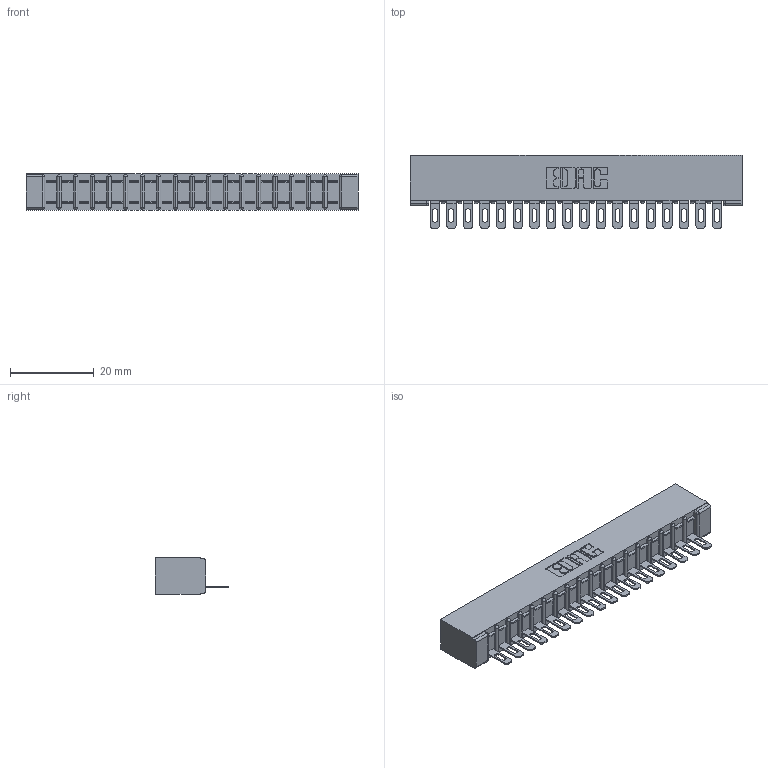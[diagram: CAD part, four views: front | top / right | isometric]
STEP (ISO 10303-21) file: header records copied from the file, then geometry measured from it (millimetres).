
FILE_DESCRIPTION (( 'STEP AP203' ), '1' );
FILE_NAME ('357-018-401-101.STEP', '2020-10-01T00:16:39', ( '' ), ( '' ), 'SwSTEP 2.0', 'SolidWorks 2020', '' );
FILE_SCHEMA (( 'CONFIG_CONTROL_DESIGN' ));
Length unit declared in the file: inch
Products named in the file (3): 357-018-401-101; 307-290-002_501; 307 Part_No Mounting Lugs
Assembly tree (19 placements, depth 2):
  357-018-401-101
    307 Part_No Mounting Lugs
    307-290-002_501  x18
Bounding box: 79.2 x 17.42 x 8.71 mm (x, y, z)
Volume: 5484.3 mm3; surface area: 10381.1 mm2
Topology: 19 solids, 19 shells, 1497 faces, 4583 edges, 3002 vertices
Faces by surface type: plane 858, cylinder 601, sphere 38
Entity records: 18906 total; most frequent: CARTESIAN_POINT 3184, ORIENTED_EDGE 3174, DIRECTION 3107, EDGE_CURVE 1587, VECTOR 1201, LINE 1201, VERTEX_POINT 1030, AXIS2_PLACEMENT_3D 953
